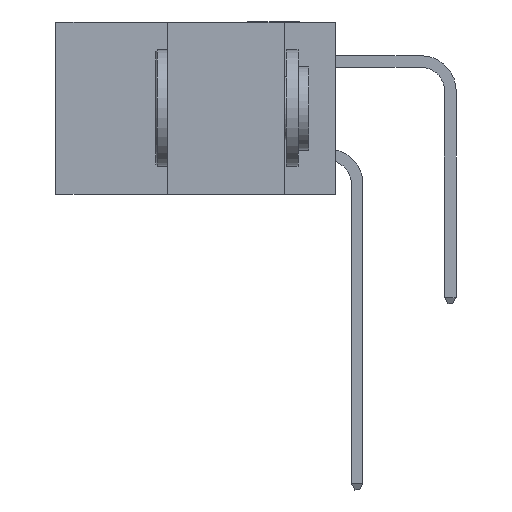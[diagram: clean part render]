
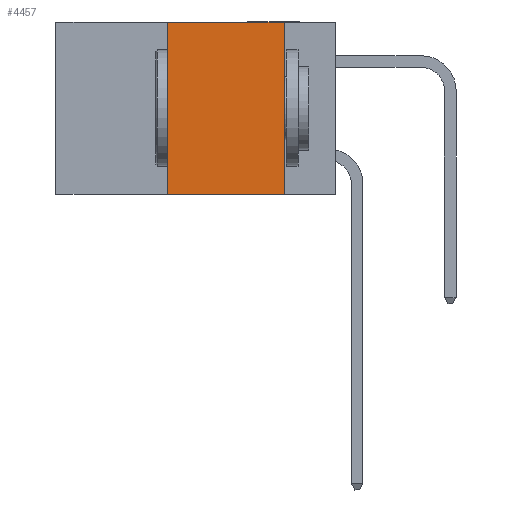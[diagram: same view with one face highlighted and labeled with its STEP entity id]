
A CAD part, left-side view. The second image highlights one B-rep face of the part: STEP entity #4457.
In plain terms, the highlighted planar face has unit normal (-1, 0, 0).
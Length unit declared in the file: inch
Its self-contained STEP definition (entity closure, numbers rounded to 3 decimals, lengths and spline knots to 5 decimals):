
#270 = ORIENTED_EDGE ( 'NONE', *, *, #3352, .F. ) ;
#384 = DIRECTION ( 'NONE',  ( 0., 0., -1. ) ) ;
#442 = VERTEX_POINT ( 'NONE', #851 ) ;
#773 = CARTESIAN_POINT ( 'NONE',  ( 0., 0.6, 0. ) ) ;
#851 = CARTESIAN_POINT ( 'NONE',  ( 0., 0.11, 0. ) ) ;
#1269 = VECTOR ( 'NONE', #1765, 39.37008 ) ;
#1299 = DIRECTION ( 'NONE',  ( 0., 0., -1. ) ) ;
#1544 = DIRECTION ( 'NONE',  ( 1., 0., 0. ) ) ;
#1707 = LINE ( 'NONE', #6328, #12367 ) ;
#1765 = DIRECTION ( 'NONE',  ( 0., 0., 1. ) ) ;
#3352 = EDGE_CURVE ( 'NONE', #8689, #9711, #3843, .T. ) ;
#3552 = VECTOR ( 'NONE', #10007, 39.37008 ) ;
#3583 = EDGE_LOOP ( 'NONE', ( #8354, #9917, #270, #12882 ) ) ;
#3775 = EDGE_CURVE ( 'NONE', #8689, #5200, #9137, .T. ) ;
#3843 = LINE ( 'NONE', #11140, #1269 ) ;
#4457 = ADVANCED_FACE ( 'NONE', ( #11887 ), #7664, .F. ) ;
#4667 = DIRECTION ( 'NONE',  ( 0., -1., 0. ) ) ;
#5200 = VERTEX_POINT ( 'NONE', #8814 ) ;
#6328 = CARTESIAN_POINT ( 'NONE',  ( 0., 0.11, 0. ) ) ;
#6821 = CARTESIAN_POINT ( 'NONE',  ( 0., 0.6, -0.37 ) ) ;
#7592 = EDGE_CURVE ( 'NONE', #442, #5200, #1707, .T. ) ;
#7614 = CARTESIAN_POINT ( 'NONE',  ( 0., 0.6, 0. ) ) ;
#7664 = PLANE ( 'NONE',  #12069 ) ;
#7821 = CARTESIAN_POINT ( 'NONE',  ( 0., 0.36, -0.37 ) ) ;
#8354 = ORIENTED_EDGE ( 'NONE', *, *, #7592, .F. ) ;
#8536 = LINE ( 'NONE', #773, #3552 ) ;
#8689 = VERTEX_POINT ( 'NONE', #7821 ) ;
#8814 = CARTESIAN_POINT ( 'NONE',  ( 0., 0.11, -0.37 ) ) ;
#9137 = LINE ( 'NONE', #6821, #11238 ) ;
#9711 = VERTEX_POINT ( 'NONE', #10916 ) ;
#9917 = ORIENTED_EDGE ( 'NONE', *, *, #10682, .F. ) ;
#10007 = DIRECTION ( 'NONE',  ( 0., -1., 0. ) ) ;
#10682 = EDGE_CURVE ( 'NONE', #9711, #442, #8536, .T. ) ;
#10916 = CARTESIAN_POINT ( 'NONE',  ( 0., 0.36, 0. ) ) ;
#11140 = CARTESIAN_POINT ( 'NONE',  ( 0., 0.36, 0. ) ) ;
#11238 = VECTOR ( 'NONE', #4667, 39.37008 ) ;
#11887 = FACE_OUTER_BOUND ( 'NONE', #3583, .T. ) ;
#12069 = AXIS2_PLACEMENT_3D ( 'NONE', #7614, #1544, #384 ) ;
#12367 = VECTOR ( 'NONE', #1299, 39.37008 ) ;
#12882 = ORIENTED_EDGE ( 'NONE', *, *, #3775, .T. ) ;
